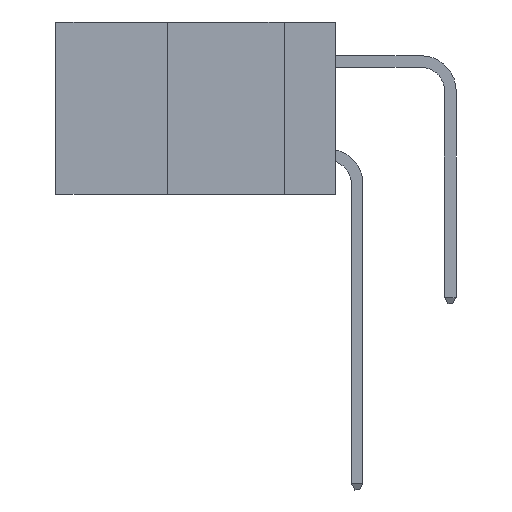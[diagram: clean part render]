
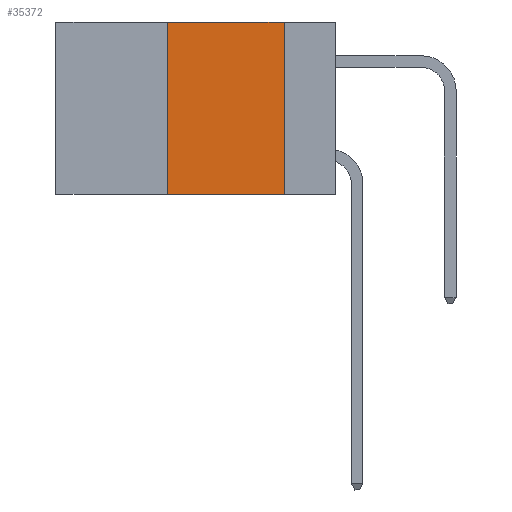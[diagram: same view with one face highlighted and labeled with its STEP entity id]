
A CAD part, left-side view. The second image highlights one B-rep face of the part: STEP entity #35372.
In plain terms, the highlighted planar face has unit normal (-1, 0, 0).
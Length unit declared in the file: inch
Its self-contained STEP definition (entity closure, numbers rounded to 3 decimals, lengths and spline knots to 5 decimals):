
#847 = VECTOR ( 'NONE', #29668, 39.37008 ) ;
#3156 = ORIENTED_EDGE ( 'NONE', *, *, #36249, .F. ) ;
#3549 = VECTOR ( 'NONE', #7702, 39.37008 ) ;
#4717 = LINE ( 'NONE', #17211, #847 ) ;
#4861 = PLANE ( 'NONE',  #9331 ) ;
#6924 = CARTESIAN_POINT ( 'NONE',  ( 0., 0.11, -0.37 ) ) ;
#6931 = EDGE_CURVE ( 'NONE', #23059, #19718, #23249, .T. ) ;
#7702 = DIRECTION ( 'NONE',  ( 0., 0., 1. ) ) ;
#7737 = FACE_OUTER_BOUND ( 'NONE', #18091, .T. ) ;
#9331 = AXIS2_PLACEMENT_3D ( 'NONE', #20233, #26153, #17165 ) ;
#13640 = CARTESIAN_POINT ( 'NONE',  ( 0., 0.36, 0. ) ) ;
#14213 = EDGE_CURVE ( 'NONE', #21771, #33932, #4717, .T. ) ;
#16452 = CARTESIAN_POINT ( 'NONE',  ( 0., 0.6, -0.37 ) ) ;
#16861 = CARTESIAN_POINT ( 'NONE',  ( 0., 0.36, -0.37 ) ) ;
#17165 = DIRECTION ( 'NONE',  ( 0., 0., -1. ) ) ;
#17211 = CARTESIAN_POINT ( 'NONE',  ( 0., 0.11, 0. ) ) ;
#18091 = EDGE_LOOP ( 'NONE', ( #27521, #3156, #26053, #36083 ) ) ;
#19718 = VERTEX_POINT ( 'NONE', #37452 ) ;
#20233 = CARTESIAN_POINT ( 'NONE',  ( 0., 0.6, 0. ) ) ;
#21771 = VERTEX_POINT ( 'NONE', #32592 ) ;
#22069 = DIRECTION ( 'NONE',  ( 0., -1., 0. ) ) ;
#22991 = CARTESIAN_POINT ( 'NONE',  ( 0., 0.6, 0. ) ) ;
#23059 = VERTEX_POINT ( 'NONE', #16861 ) ;
#23249 = LINE ( 'NONE', #13640, #3549 ) ;
#24411 = VECTOR ( 'NONE', #29532, 39.37008 ) ;
#26053 = ORIENTED_EDGE ( 'NONE', *, *, #6931, .F. ) ;
#26153 = DIRECTION ( 'NONE',  ( 1., 0., 0. ) ) ;
#26993 = EDGE_CURVE ( 'NONE', #23059, #33932, #28006, .T. ) ;
#27274 = VECTOR ( 'NONE', #22069, 39.37008 ) ;
#27521 = ORIENTED_EDGE ( 'NONE', *, *, #14213, .F. ) ;
#28006 = LINE ( 'NONE', #16452, #27274 ) ;
#28933 = LINE ( 'NONE', #22991, #24411 ) ;
#29532 = DIRECTION ( 'NONE',  ( 0., -1., 0. ) ) ;
#29668 = DIRECTION ( 'NONE',  ( 0., 0., -1. ) ) ;
#32592 = CARTESIAN_POINT ( 'NONE',  ( 0., 0.11, 0. ) ) ;
#33932 = VERTEX_POINT ( 'NONE', #6924 ) ;
#35372 = ADVANCED_FACE ( 'NONE', ( #7737 ), #4861, .F. ) ;
#36083 = ORIENTED_EDGE ( 'NONE', *, *, #26993, .T. ) ;
#36249 = EDGE_CURVE ( 'NONE', #19718, #21771, #28933, .T. ) ;
#37452 = CARTESIAN_POINT ( 'NONE',  ( 0., 0.36, 0. ) ) ;
